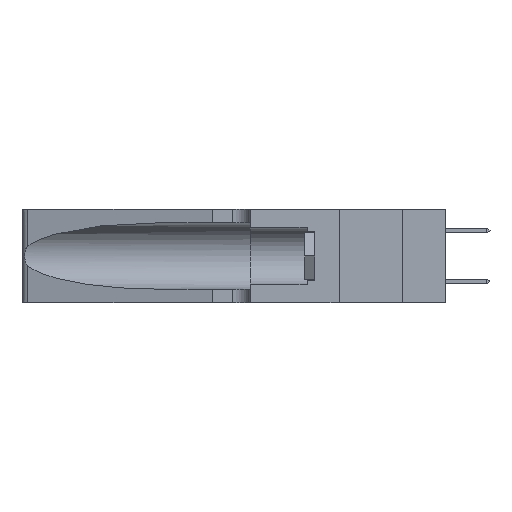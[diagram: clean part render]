
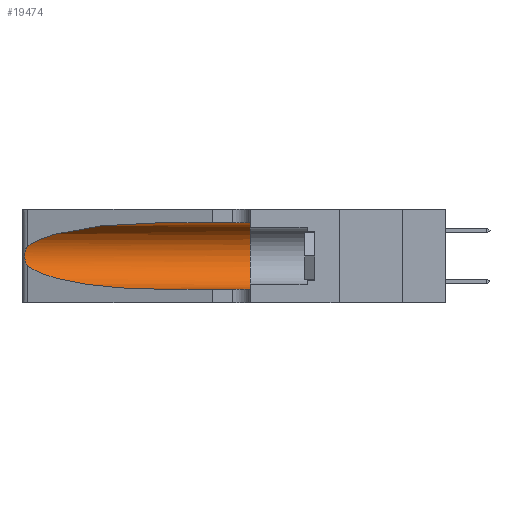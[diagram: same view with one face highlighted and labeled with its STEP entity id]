
A CAD part, left-side view. The second image highlights one B-rep face of the part: STEP entity #19474.
In plain terms, the highlighted cylindrical face has radius 3.308 mm (diameter 6.617 mm), a partial arc.
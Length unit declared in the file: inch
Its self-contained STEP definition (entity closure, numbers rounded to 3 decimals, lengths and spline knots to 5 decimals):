
#54 =( BOUNDED_CURVE ( )  B_SPLINE_CURVE ( 3, ( #9522, #18532, #11021, #1804 ),
 .UNSPECIFIED., .F., .F. ) 
 B_SPLINE_CURVE_WITH_KNOTS ( ( 4, 4 ),
 ( 1.5708, 2.84003 ),
 .UNSPECIFIED. ) 
 CURVE ( )  GEOMETRIC_REPRESENTATION_ITEM ( )  RATIONAL_B_SPLINE_CURVE ( ( 1., 0.87, 0.87, 1. ) ) 
 REPRESENTATION_ITEM ( '' )  );
#392 = CARTESIAN_POINT ( 'NONE',  ( 0.1305, 1.61858, 0.185 ) ) ;
#867 = LINE ( 'NONE', #14455, #12178 ) ;
#1451 = CARTESIAN_POINT ( 'NONE',  ( 0.25856, 1.23593, 0.16098 ) ) ;
#1512 = VERTEX_POINT ( 'NONE', #11741 ) ;
#1694 = VERTEX_POINT ( 'NONE', #4871 ) ;
#1804 = CARTESIAN_POINT ( 'NONE',  ( 0.25487, 1.22718, 0.22369 ) ) ;
#1828 = DIRECTION ( 'NONE',  ( 0., 1., 0. ) ) ;
#2997 = CARTESIAN_POINT ( 'NONE',  ( 0.1305, 0.35, 0.05475 ) ) ;
#3023 = CARTESIAN_POINT ( 'NONE',  ( 0.25639, 1.23186, 0.15144 ) ) ;
#3127 = VECTOR ( 'NONE', #7754, 39.37008 ) ;
#3238 = CARTESIAN_POINT ( 'NONE',  ( 0.1305, 0.72297, 0.05475 ) ) ;
#3850 = DIRECTION ( 'NONE',  ( 0., -1., 0. ) ) ;
#3903 = EDGE_LOOP ( 'NONE', ( #8844, #16816, #5270, #13311, #9761, #17765 ) ) ;
#4003 = VERTEX_POINT ( 'NONE', #3238 ) ;
#4639 = CARTESIAN_POINT ( 'NONE',  ( 0.25487, 1.22718, 0.14631 ) ) ;
#4739 = CARTESIAN_POINT ( 'NONE',  ( 0.2373, 1.15595, 0.08982 ) ) ;
#4769 = CARTESIAN_POINT ( 'NONE',  ( 0.1305, 0.35, 0.31525 ) ) ;
#4871 = CARTESIAN_POINT ( 'NONE',  ( 0.25487, 1.22718, 0.14631 ) ) ;
#5101 = DIRECTION ( 'NONE',  ( 0., -1., 0. ) ) ;
#5270 = ORIENTED_EDGE ( 'NONE', *, *, #12697, .T. ) ;
#6073 = CARTESIAN_POINT ( 'NONE',  ( 0.25487, 1.22718, 0.22369 ) ) ;
#6086 = AXIS2_PLACEMENT_3D ( 'NONE', #11048, #1828, #12568 ) ;
#6144 = CARTESIAN_POINT ( 'NONE',  ( 0.25639, 1.23184, 0.21858 ) ) ;
#6166 = CARTESIAN_POINT ( 'NONE',  ( 0.1305, 1.61858, 0.05475 ) ) ;
#6368 = CARTESIAN_POINT ( 'NONE',  ( 0.1305, 0.72297, 0.05475 ) ) ;
#6862 = CYLINDRICAL_SURFACE ( 'NONE', #13148, 0.13025 ) ;
#7292 = LINE ( 'NONE', #6166, #3127 ) ;
#7671 = CARTESIAN_POINT ( 'NONE',  ( 0.25854, 1.2359, 0.20912 ) ) ;
#7754 = DIRECTION ( 'NONE',  ( 0., -1., 0. ) ) ;
#8343 = VERTEX_POINT ( 'NONE', #4769 ) ;
#8844 = ORIENTED_EDGE ( 'NONE', *, *, #18238, .T. ) ;
#9177 = CARTESIAN_POINT ( 'NONE',  ( 0.26075, 1.23896, 0.19203 ) ) ;
#9327 = CARTESIAN_POINT ( 'NONE',  ( 0.25487, 1.22718, 0.14631 ) ) ;
#9522 = CARTESIAN_POINT ( 'NONE',  ( 0.1305, 0.72297, 0.31525 ) ) ;
#9761 = ORIENTED_EDGE ( 'NONE', *, *, #19421, .F. ) ;
#10677 = CARTESIAN_POINT ( 'NONE',  ( 0.26017, 1.23833, 0.17102 ) ) ;
#10961 = B_SPLINE_CURVE_WITH_KNOTS ( 'NONE', 3,
 ( #6073, #12118, #6144, #16640, #7671, #18189, #9177, #19669, #10677, #1451, #12186, #3023, #13703, #4639 ),
 .UNSPECIFIED., .F., .F.,
 ( 4, 2, 2, 2, 2, 2, 4 ),
 ( 0., 0.00027, 0.00053, 0.00107, 0.0016, 0.00187, 0.00214 ),
 .UNSPECIFIED. ) ;
#11021 = CARTESIAN_POINT ( 'NONE',  ( 0.2373, 1.15595, 0.28018 ) ) ;
#11048 = CARTESIAN_POINT ( 'NONE',  ( 0.1305, 0.35, 0.185 ) ) ;
#11181 = DIRECTION ( 'NONE',  ( 0., 0., -1. ) ) ;
#11741 = CARTESIAN_POINT ( 'NONE',  ( 0.25487, 1.22718, 0.22369 ) ) ;
#12118 = CARTESIAN_POINT ( 'NONE',  ( 0.25555, 1.22994, 0.2215 ) ) ;
#12178 = VECTOR ( 'NONE', #3850, 39.37008 ) ;
#12186 = CARTESIAN_POINT ( 'NONE',  ( 0.25789, 1.23486, 0.15765 ) ) ;
#12273 = CIRCLE ( 'NONE', #6086, 0.13025 ) ;
#12480 =( BOUNDED_CURVE ( )  B_SPLINE_CURVE ( 3, ( #9327, #4739, #15342, #6368 ),
 .UNSPECIFIED., .F., .F. ) 
 B_SPLINE_CURVE_WITH_KNOTS ( ( 4, 4 ),
 ( 3.44316, 4.71239 ),
 .UNSPECIFIED. ) 
 CURVE ( )  GEOMETRIC_REPRESENTATION_ITEM ( )  RATIONAL_B_SPLINE_CURVE ( ( 1., 0.87, 0.87, 1. ) ) 
 REPRESENTATION_ITEM ( '' )  );
#12568 = DIRECTION ( 'NONE',  ( 0., 0., 1. ) ) ;
#12697 = EDGE_CURVE ( 'NONE', #1694, #4003, #12480, .T. ) ;
#13148 = AXIS2_PLACEMENT_3D ( 'NONE', #392, #5101, #11181 ) ;
#13311 = ORIENTED_EDGE ( 'NONE', *, *, #14119, .T. ) ;
#13703 = CARTESIAN_POINT ( 'NONE',  ( 0.25555, 1.22993, 0.14849 ) ) ;
#14119 = EDGE_CURVE ( 'NONE', #4003, #18098, #7292, .T. ) ;
#14455 = CARTESIAN_POINT ( 'NONE',  ( 0.1305, 1.61858, 0.31525 ) ) ;
#14834 = FACE_OUTER_BOUND ( 'NONE', #3903, .T. ) ;
#14970 = EDGE_CURVE ( 'NONE', #16028, #8343, #867, .T. ) ;
#15342 = CARTESIAN_POINT ( 'NONE',  ( 0.18966, 0.96281, 0.05475 ) ) ;
#16028 = VERTEX_POINT ( 'NONE', #18334 ) ;
#16640 = CARTESIAN_POINT ( 'NONE',  ( 0.25787, 1.23484, 0.2124 ) ) ;
#16816 = ORIENTED_EDGE ( 'NONE', *, *, #17419, .T. ) ;
#17419 = EDGE_CURVE ( 'NONE', #1512, #1694, #10961, .T. ) ;
#17765 = ORIENTED_EDGE ( 'NONE', *, *, #14970, .F. ) ;
#18098 = VERTEX_POINT ( 'NONE', #2997 ) ;
#18189 = CARTESIAN_POINT ( 'NONE',  ( 0.26018, 1.23835, 0.19895 ) ) ;
#18238 = EDGE_CURVE ( 'NONE', #16028, #1512, #54, .T. ) ;
#18334 = CARTESIAN_POINT ( 'NONE',  ( 0.1305, 0.72297, 0.31525 ) ) ;
#18532 = CARTESIAN_POINT ( 'NONE',  ( 0.18966, 0.96281, 0.31525 ) ) ;
#19421 = EDGE_CURVE ( 'NONE', #8343, #18098, #12273, .T. ) ;
#19474 = ADVANCED_FACE ( 'NONE', ( #14834 ), #6862, .F. ) ;
#19669 = CARTESIAN_POINT ( 'NONE',  ( 0.26075, 1.23896, 0.178 ) ) ;
